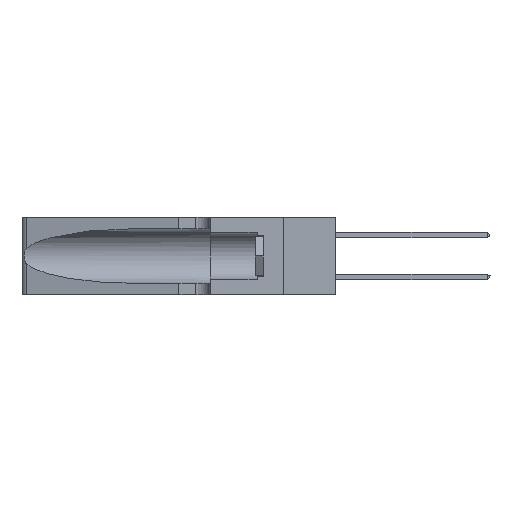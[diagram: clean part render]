
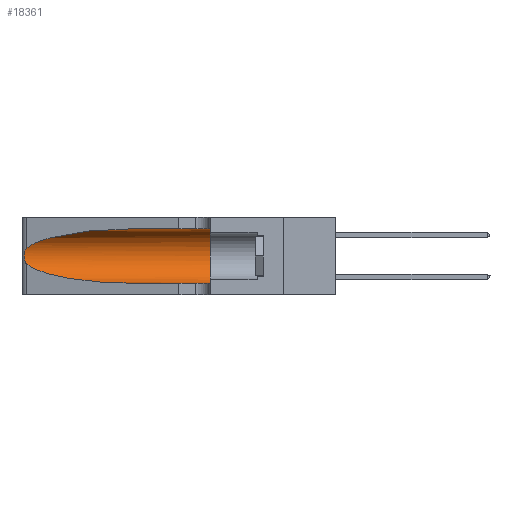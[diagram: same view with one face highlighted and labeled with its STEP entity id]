
A CAD part, left-side view. The second image highlights one B-rep face of the part: STEP entity #18361.
In plain terms, the highlighted cylindrical face has radius 3.308 mm (diameter 6.617 mm), a partial arc.
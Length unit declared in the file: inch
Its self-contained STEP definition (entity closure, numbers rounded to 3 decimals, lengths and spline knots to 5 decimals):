
#43 = CARTESIAN_POINT ( 'NONE',  ( 0.1305, 0.35, 0.05475 ) ) ;
#53 = VECTOR ( 'NONE', #506, 39.37008 ) ;
#506 = DIRECTION ( 'NONE',  ( 0., -1., 0. ) ) ;
#523 = EDGE_CURVE ( 'NONE', #6284, #42195, #3062, .T. ) ;
#2172 = CARTESIAN_POINT ( 'NONE',  ( 0.26075, 1.23896, 0.178 ) ) ;
#2482 = CARTESIAN_POINT ( 'NONE',  ( 0.26075, 1.23896, 0.19203 ) ) ;
#3062 =( BOUNDED_CURVE ( )  B_SPLINE_CURVE ( 3, ( #34543, #30839, #34702, #45633 ),
 .UNSPECIFIED., .F., .T. ) 
 B_SPLINE_CURVE_WITH_KNOTS ( ( 4, 4 ),
 ( 1.5708, 2.84003 ),
 .UNSPECIFIED. ) 
 CURVE ( )  GEOMETRIC_REPRESENTATION_ITEM ( )  RATIONAL_B_SPLINE_CURVE ( ( 1., 0.87, 0.87, 1. ) ) 
 REPRESENTATION_ITEM ( '' )  );
#3254 = CARTESIAN_POINT ( 'NONE',  ( 0.1305, 0.72297, 0.31525 ) ) ;
#3533 = CARTESIAN_POINT ( 'NONE',  ( 0.25487, 1.22718, 0.14631 ) ) ;
#3990 = ORIENTED_EDGE ( 'NONE', *, *, #15700, .T. ) ;
#4057 = VERTEX_POINT ( 'NONE', #3533 ) ;
#5166 = CARTESIAN_POINT ( 'NONE',  ( 0.1305, 0.72297, 0.05475 ) ) ;
#5849 = CARTESIAN_POINT ( 'NONE',  ( 0.26017, 1.23833, 0.17102 ) ) ;
#6284 = VERTEX_POINT ( 'NONE', #3254 ) ;
#8546 = CARTESIAN_POINT ( 'NONE',  ( 0.1305, 1.61858, 0.05475 ) ) ;
#12404 = DIRECTION ( 'NONE',  ( 0., -1., 0. ) ) ;
#14416 = AXIS2_PLACEMENT_3D ( 'NONE', #17874, #14501, #21714 ) ;
#14437 = CARTESIAN_POINT ( 'NONE',  ( 0.1305, 1.61858, 0.185 ) ) ;
#14501 = DIRECTION ( 'NONE',  ( 0., 1., 0. ) ) ;
#14979 = CARTESIAN_POINT ( 'NONE',  ( 0.1305, 0.35, 0.31525 ) ) ;
#14992 = FACE_OUTER_BOUND ( 'NONE', #46573, .T. ) ;
#15302 = LINE ( 'NONE', #8546, #35971 ) ;
#15423 = VERTEX_POINT ( 'NONE', #14979 ) ;
#15700 = EDGE_CURVE ( 'NONE', #29272, #36860, #15302, .T. ) ;
#16556 = CARTESIAN_POINT ( 'NONE',  ( 0.25639, 1.23186, 0.15144 ) ) ;
#17663 = DIRECTION ( 'NONE',  ( 0., -1., 0. ) ) ;
#17705 = EDGE_CURVE ( 'NONE', #42195, #4057, #35034, .T. ) ;
#17874 = CARTESIAN_POINT ( 'NONE',  ( 0.1305, 0.35, 0.185 ) ) ;
#18361 = ADVANCED_FACE ( 'NONE', ( #14992 ), #39095, .F. ) ;
#18633 = EDGE_CURVE ( 'NONE', #6284, #15423, #36745, .T. ) ;
#20254 = CARTESIAN_POINT ( 'NONE',  ( 0.25856, 1.23593, 0.16098 ) ) ;
#20563 = CARTESIAN_POINT ( 'NONE',  ( 0.25487, 1.22718, 0.14631 ) ) ;
#21151 = ORIENTED_EDGE ( 'NONE', *, *, #523, .T. ) ;
#21714 = DIRECTION ( 'NONE',  ( 0., 0., 1. ) ) ;
#22436 = CARTESIAN_POINT ( 'NONE',  ( 0.1305, 1.61858, 0.31525 ) ) ;
#23136 = ORIENTED_EDGE ( 'NONE', *, *, #30168, .T. ) ;
#23940 = CARTESIAN_POINT ( 'NONE',  ( 0.25639, 1.23184, 0.21858 ) ) ;
#24102 = CARTESIAN_POINT ( 'NONE',  ( 0.25854, 1.2359, 0.20912 ) ) ;
#26685 = AXIS2_PLACEMENT_3D ( 'NONE', #14437, #17663, #32538 ) ;
#27454 = CARTESIAN_POINT ( 'NONE',  ( 0.25787, 1.23484, 0.2124 ) ) ;
#27785 = CARTESIAN_POINT ( 'NONE',  ( 0.26018, 1.23835, 0.19895 ) ) ;
#28111 = CARTESIAN_POINT ( 'NONE',  ( 0.18966, 0.96281, 0.05475 ) ) ;
#29272 = VERTEX_POINT ( 'NONE', #5166 ) ;
#30168 = EDGE_CURVE ( 'NONE', #4057, #29272, #43564, .T. ) ;
#30305 = EDGE_CURVE ( 'NONE', #15423, #36860, #35390, .T. ) ;
#30485 = ORIENTED_EDGE ( 'NONE', *, *, #17705, .T. ) ;
#30839 = CARTESIAN_POINT ( 'NONE',  ( 0.18966, 0.96281, 0.31525 ) ) ;
#31980 = ORIENTED_EDGE ( 'NONE', *, *, #18633, .F. ) ;
#32538 = DIRECTION ( 'NONE',  ( 0., 0., -1. ) ) ;
#34543 = CARTESIAN_POINT ( 'NONE',  ( 0.1305, 0.72297, 0.31525 ) ) ;
#34702 = CARTESIAN_POINT ( 'NONE',  ( 0.2373, 1.15595, 0.28018 ) ) ;
#35034 = B_SPLINE_CURVE_WITH_KNOTS ( 'NONE', 3,
 ( #35314, #42523, #23940, #27454, #24102, #27785, #2482, #2172, #5849, #20254, #35162, #16556, #38840, #20563 ),
 .UNSPECIFIED., .F., .F.,
 ( 4, 2, 2, 2, 2, 2, 4 ),
 ( 0., 0.00027, 0.00053, 0.00107, 0.0016, 0.00187, 0.00214 ),
 .UNSPECIFIED. ) ;
#35162 = CARTESIAN_POINT ( 'NONE',  ( 0.25789, 1.23486, 0.15765 ) ) ;
#35314 = CARTESIAN_POINT ( 'NONE',  ( 0.25487, 1.22718, 0.22369 ) ) ;
#35390 = CIRCLE ( 'NONE', #14416, 0.13025 ) ;
#35679 = CARTESIAN_POINT ( 'NONE',  ( 0.1305, 0.72297, 0.05475 ) ) ;
#35971 = VECTOR ( 'NONE', #12404, 39.37008 ) ;
#36745 = LINE ( 'NONE', #22436, #53 ) ;
#36860 = VERTEX_POINT ( 'NONE', #43 ) ;
#38840 = CARTESIAN_POINT ( 'NONE',  ( 0.25555, 1.22993, 0.14849 ) ) ;
#39095 = CYLINDRICAL_SURFACE ( 'NONE', #26685, 0.13025 ) ;
#39219 = CARTESIAN_POINT ( 'NONE',  ( 0.25487, 1.22718, 0.14631 ) ) ;
#42195 = VERTEX_POINT ( 'NONE', #42388 ) ;
#42388 = CARTESIAN_POINT ( 'NONE',  ( 0.25487, 1.22718, 0.22369 ) ) ;
#42523 = CARTESIAN_POINT ( 'NONE',  ( 0.25555, 1.22994, 0.2215 ) ) ;
#43564 =( BOUNDED_CURVE ( )  B_SPLINE_CURVE ( 3, ( #39219, #46128, #28111, #35679 ),
 .UNSPECIFIED., .F., .F. ) 
 B_SPLINE_CURVE_WITH_KNOTS ( ( 4, 4 ),
 ( 3.44316, 4.71239 ),
 .UNSPECIFIED. ) 
 CURVE ( )  GEOMETRIC_REPRESENTATION_ITEM ( )  RATIONAL_B_SPLINE_CURVE ( ( 1., 0.87, 0.87, 1. ) ) 
 REPRESENTATION_ITEM ( '' )  );
#45633 = CARTESIAN_POINT ( 'NONE',  ( 0.25487, 1.22718, 0.22369 ) ) ;
#46128 = CARTESIAN_POINT ( 'NONE',  ( 0.2373, 1.15595, 0.08982 ) ) ;
#46573 = EDGE_LOOP ( 'NONE', ( #21151, #30485, #23136, #3990, #46895, #31980 ) ) ;
#46895 = ORIENTED_EDGE ( 'NONE', *, *, #30305, .F. ) ;
